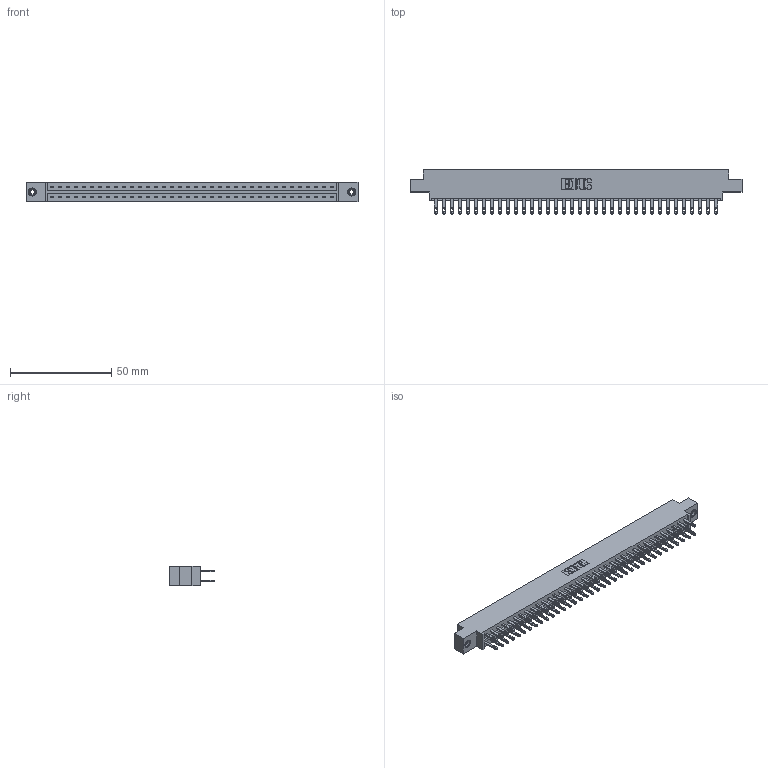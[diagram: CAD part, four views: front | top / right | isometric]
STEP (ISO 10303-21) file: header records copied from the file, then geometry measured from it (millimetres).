
FILE_DESCRIPTION (( 'STEP AP203' ), '1' );
FILE_NAME ('333-072-500-808.STEP', '2018-08-04T15:58:53', ( '' ), ( '' ), 'SwSTEP 2.0', 'SolidWorks 2016', '' );
FILE_SCHEMA (( 'CONFIG_CONTROL_DESIGN' ));
Length unit declared in the file: inch
Products named in the file (4): 345-250-001_345-250-003-102; 333-072-500-808; 333 Part_Offset - .156 Dia - TI; 345-292-001_345-293-100
Assembly tree (75 placements, depth 2):
  333-072-500-808
    333 Part_Offset - .156 Dia - TI
    345-292-001_345-293-100  x72
    345-250-001_345-250-003-102  x2
Bounding box: 164.19 x 21.85 x 9.4 mm (x, y, z)
Volume: 16692 mm3; surface area: 20704.5 mm2
Topology: 75 solids, 75 shells, 3634 faces, 11043 edges, 7354 vertices
Faces by surface type: plane 2266, cylinder 1352, cone 12, torus 4
Entity records: 25184 total; most frequent: CARTESIAN_POINT 4165, ORIENTED_EDGE 4094, DIRECTION 3601, EDGE_CURVE 2047, LINE 1895, VECTOR 1895, VERTEX_POINT 1360, AXIS2_PLACEMENT_3D 853
